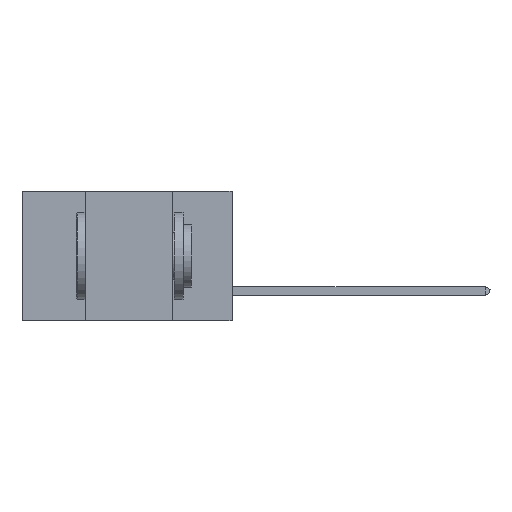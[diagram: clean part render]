
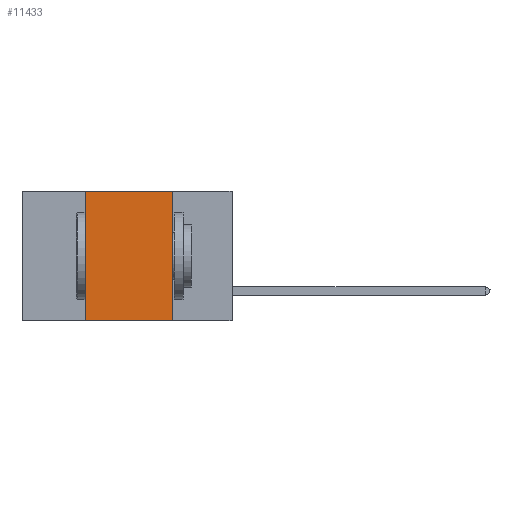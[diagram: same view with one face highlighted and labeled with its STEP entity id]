
A CAD part, left-side view. The second image highlights one B-rep face of the part: STEP entity #11433.
In plain terms, the highlighted planar face has unit normal (-1, 0, 0).
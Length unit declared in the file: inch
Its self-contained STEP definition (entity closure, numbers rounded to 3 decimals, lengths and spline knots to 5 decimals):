
#1047 = ORIENTED_EDGE ( 'NONE', *, *, #22071, .T. ) ;
#1049 = LINE ( 'NONE', #28161, #24325 ) ;
#1323 = VECTOR ( 'NONE', #12181, 39.37008 ) ;
#3691 = DIRECTION ( 'NONE',  ( 0., 0., -1. ) ) ;
#3995 = CARTESIAN_POINT ( 'NONE',  ( 0., 0.17, 0. ) ) ;
#4780 = CARTESIAN_POINT ( 'NONE',  ( 0., 0.6, -0.37 ) ) ;
#5087 = CARTESIAN_POINT ( 'NONE',  ( 0., 0.17, 0. ) ) ;
#5702 = DIRECTION ( 'NONE',  ( 1., 0., 0. ) ) ;
#6787 = CARTESIAN_POINT ( 'NONE',  ( 0., 0.42, -0.37 ) ) ;
#6862 = DIRECTION ( 'NONE',  ( 0., -1., 0. ) ) ;
#7991 = LINE ( 'NONE', #5087, #1323 ) ;
#8232 = AXIS2_PLACEMENT_3D ( 'NONE', #19266, #5702, #3691 ) ;
#8607 = DIRECTION ( 'NONE',  ( 0., 0., 1. ) ) ;
#8771 = VECTOR ( 'NONE', #8607, 39.37008 ) ;
#10021 = CARTESIAN_POINT ( 'NONE',  ( 0., 0.17, -0.37 ) ) ;
#10631 = EDGE_CURVE ( 'NONE', #27301, #17349, #21805, .T. ) ;
#10886 = FACE_OUTER_BOUND ( 'NONE', #25404, .T. ) ;
#11433 = ADVANCED_FACE ( 'NONE', ( #10886 ), #12827, .F. ) ;
#11563 = ORIENTED_EDGE ( 'NONE', *, *, #22744, .F. ) ;
#11908 = ORIENTED_EDGE ( 'NONE', *, *, #21619, .F. ) ;
#12181 = DIRECTION ( 'NONE',  ( 0., 0., -1. ) ) ;
#12827 = PLANE ( 'NONE',  #8232 ) ;
#12830 = ORIENTED_EDGE ( 'NONE', *, *, #10631, .F. ) ;
#14784 = DIRECTION ( 'NONE',  ( 0., -1., 0. ) ) ;
#17349 = VERTEX_POINT ( 'NONE', #25899 ) ;
#19266 = CARTESIAN_POINT ( 'NONE',  ( 0., 0.6, 0. ) ) ;
#19366 = LINE ( 'NONE', #4780, #26373 ) ;
#21528 = VERTEX_POINT ( 'NONE', #10021 ) ;
#21619 = EDGE_CURVE ( 'NONE', #17349, #26721, #1049, .T. ) ;
#21805 = LINE ( 'NONE', #28920, #8771 ) ;
#22071 = EDGE_CURVE ( 'NONE', #27301, #21528, #19366, .T. ) ;
#22744 = EDGE_CURVE ( 'NONE', #26721, #21528, #7991, .T. ) ;
#24325 = VECTOR ( 'NONE', #14784, 39.37008 ) ;
#25404 = EDGE_LOOP ( 'NONE', ( #11563, #11908, #12830, #1047 ) ) ;
#25899 = CARTESIAN_POINT ( 'NONE',  ( 0., 0.42, 0. ) ) ;
#26373 = VECTOR ( 'NONE', #6862, 39.37008 ) ;
#26721 = VERTEX_POINT ( 'NONE', #3995 ) ;
#27301 = VERTEX_POINT ( 'NONE', #6787 ) ;
#28161 = CARTESIAN_POINT ( 'NONE',  ( 0., 0.6, 0. ) ) ;
#28920 = CARTESIAN_POINT ( 'NONE',  ( 0., 0.42, 0. ) ) ;
